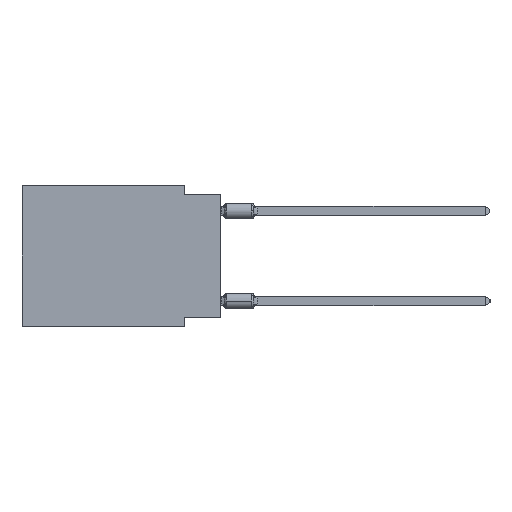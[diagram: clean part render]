
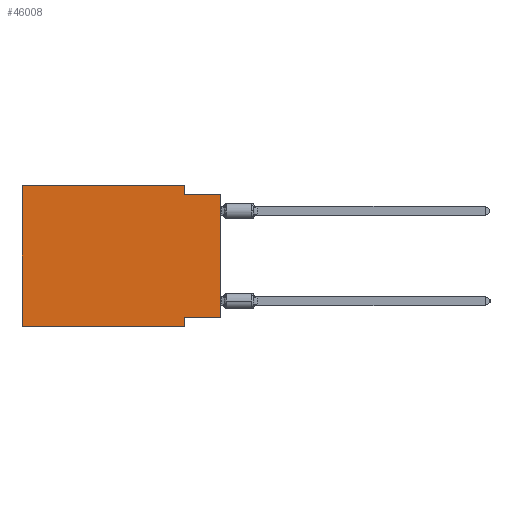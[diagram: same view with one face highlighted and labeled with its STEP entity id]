
A CAD part, left-side view. The second image highlights one B-rep face of the part: STEP entity #46008.
In plain terms, the highlighted planar face has unit normal (-1, 0, 0).
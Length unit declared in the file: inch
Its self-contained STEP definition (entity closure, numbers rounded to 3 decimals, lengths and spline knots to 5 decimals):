
#2903 = ORIENTED_EDGE ( 'NONE', *, *, #40822, .F. ) ;
#3469 = CARTESIAN_POINT ( 'NONE',  ( 0., 0.55, 0. ) ) ;
#4166 = FACE_OUTER_BOUND ( 'NONE', #18774, .T. ) ;
#4481 = DIRECTION ( 'NONE',  ( 0., 0., -1. ) ) ;
#4513 = VECTOR ( 'NONE', #4481, 39.37008 ) ;
#4642 = DIRECTION ( 'NONE',  ( 1., 0., 0. ) ) ;
#7494 = VECTOR ( 'NONE', #23106, 39.37008 ) ;
#8204 = ORIENTED_EDGE ( 'NONE', *, *, #19645, .F. ) ;
#9573 = VECTOR ( 'NONE', #20719, 39.37008 ) ;
#10914 = VERTEX_POINT ( 'NONE', #21564 ) ;
#11356 = VERTEX_POINT ( 'NONE', #21510 ) ;
#11759 = ORIENTED_EDGE ( 'NONE', *, *, #32873, .F. ) ;
#12579 = AXIS2_PLACEMENT_3D ( 'NONE', #41570, #4642, #34531 ) ;
#12623 = CARTESIAN_POINT ( 'NONE',  ( 0., 0., -0.025 ) ) ;
#13792 = EDGE_CURVE ( 'NONE', #34206, #34398, #28498, .T. ) ;
#13850 = VECTOR ( 'NONE', #18263, 39.37008 ) ;
#16469 = EDGE_CURVE ( 'NONE', #10914, #45619, #26063, .T. ) ;
#18263 = DIRECTION ( 'NONE',  ( 0., -1., 0. ) ) ;
#18481 = LINE ( 'NONE', #29439, #41550 ) ;
#18774 = EDGE_LOOP ( 'NONE', ( #27982, #11759, #35652, #35623, #8204, #38013, #22230, #2903 ) ) ;
#19050 = VECTOR ( 'NONE', #37489, 39.37008 ) ;
#19645 = EDGE_CURVE ( 'NONE', #34206, #43659, #41630, .T. ) ;
#20719 = DIRECTION ( 'NONE',  ( 0., -1., 0. ) ) ;
#21510 = CARTESIAN_POINT ( 'NONE',  ( 0., 0., -0.365 ) ) ;
#21564 = CARTESIAN_POINT ( 'NONE',  ( 0., 0.1, 0. ) ) ;
#21909 = LINE ( 'NONE', #3469, #13850 ) ;
#22230 = ORIENTED_EDGE ( 'NONE', *, *, #36153, .F. ) ;
#23106 = DIRECTION ( 'NONE',  ( 0., 0., 1. ) ) ;
#23167 = CARTESIAN_POINT ( 'NONE',  ( 0., 0.55, 0. ) ) ;
#23550 = VERTEX_POINT ( 'NONE', #12623 ) ;
#23821 = CARTESIAN_POINT ( 'NONE',  ( 0., 0., 0. ) ) ;
#25856 = CARTESIAN_POINT ( 'NONE',  ( 0., 0.1, -0.39 ) ) ;
#26063 = LINE ( 'NONE', #40885, #19050 ) ;
#26583 = LINE ( 'NONE', #41403, #4513 ) ;
#26759 = PLANE ( 'NONE',  #12579 ) ;
#27904 = VECTOR ( 'NONE', #40697, 39.37008 ) ;
#27982 = ORIENTED_EDGE ( 'NONE', *, *, #33834, .T. ) ;
#28498 = LINE ( 'NONE', #43319, #9573 ) ;
#29439 = CARTESIAN_POINT ( 'NONE',  ( 0., 0., -0.025 ) ) ;
#29526 = LINE ( 'NONE', #45063, #27904 ) ;
#32873 = EDGE_CURVE ( 'NONE', #45619, #23550, #18481, .T. ) ;
#33834 = EDGE_CURVE ( 'NONE', #11356, #23550, #45460, .T. ) ;
#33868 = DIRECTION ( 'NONE',  ( 0., 0., 1. ) ) ;
#34206 = VERTEX_POINT ( 'NONE', #45642 ) ;
#34398 = VERTEX_POINT ( 'NONE', #25856 ) ;
#34531 = DIRECTION ( 'NONE',  ( 0., 0., -1. ) ) ;
#35623 = ORIENTED_EDGE ( 'NONE', *, *, #39976, .F. ) ;
#35652 = ORIENTED_EDGE ( 'NONE', *, *, #16469, .F. ) ;
#36153 = EDGE_CURVE ( 'NONE', #39935, #34398, #26583, .T. ) ;
#37489 = DIRECTION ( 'NONE',  ( 0., 0., -1. ) ) ;
#38013 = ORIENTED_EDGE ( 'NONE', *, *, #13792, .T. ) ;
#39326 = VECTOR ( 'NONE', #33868, 39.37008 ) ;
#39935 = VERTEX_POINT ( 'NONE', #47671 ) ;
#39976 = EDGE_CURVE ( 'NONE', #43659, #10914, #21909, .T. ) ;
#40697 = DIRECTION ( 'NONE',  ( 0., 1., 0. ) ) ;
#40822 = EDGE_CURVE ( 'NONE', #11356, #39935, #29526, .T. ) ;
#40885 = CARTESIAN_POINT ( 'NONE',  ( 0., 0.1, 0. ) ) ;
#41403 = CARTESIAN_POINT ( 'NONE',  ( 0., 0.1, -0.39 ) ) ;
#41550 = VECTOR ( 'NONE', #44256, 39.37008 ) ;
#41570 = CARTESIAN_POINT ( 'NONE',  ( 0., 0.55, 0. ) ) ;
#41630 = LINE ( 'NONE', #23167, #39326 ) ;
#43319 = CARTESIAN_POINT ( 'NONE',  ( 0., 0.55, -0.39 ) ) ;
#43659 = VERTEX_POINT ( 'NONE', #46796 ) ;
#44256 = DIRECTION ( 'NONE',  ( 0., -1., 0. ) ) ;
#45063 = CARTESIAN_POINT ( 'NONE',  ( 0., 0., -0.365 ) ) ;
#45460 = LINE ( 'NONE', #23821, #7494 ) ;
#45520 = CARTESIAN_POINT ( 'NONE',  ( 0., 0.1, -0.025 ) ) ;
#45619 = VERTEX_POINT ( 'NONE', #45520 ) ;
#45642 = CARTESIAN_POINT ( 'NONE',  ( 0., 0.55, -0.39 ) ) ;
#46008 = ADVANCED_FACE ( 'NONE', ( #4166 ), #26759, .F. ) ;
#46796 = CARTESIAN_POINT ( 'NONE',  ( 0., 0.55, 0. ) ) ;
#47671 = CARTESIAN_POINT ( 'NONE',  ( 0., 0.1, -0.365 ) ) ;
